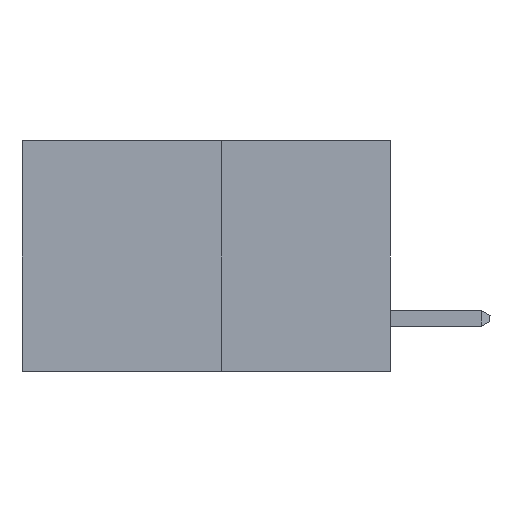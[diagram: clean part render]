
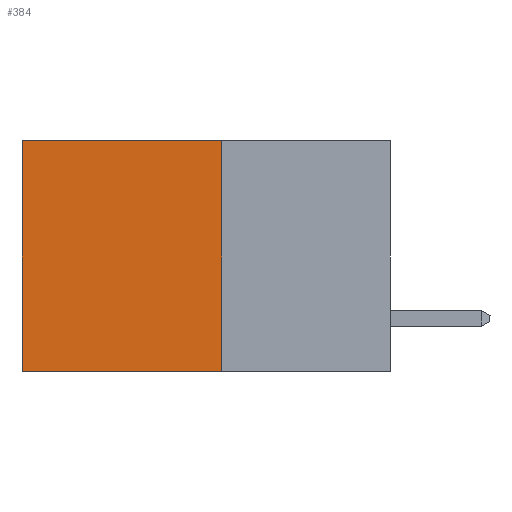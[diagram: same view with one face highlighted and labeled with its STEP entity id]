
A CAD part, left-side view. The second image highlights one B-rep face of the part: STEP entity #384.
In plain terms, the highlighted planar face has unit normal (-1, 0, 0).
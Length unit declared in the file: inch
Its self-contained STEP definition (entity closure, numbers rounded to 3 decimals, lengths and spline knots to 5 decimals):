
#384 = ADVANCED_FACE ( 'NONE', ( #8209 ), #15060, .F. ) ;
#735 = CARTESIAN_POINT ( 'NONE',  ( 0.277, 0.27, -0.37 ) ) ;
#890 = DIRECTION ( 'NONE',  ( 0., 0., -1. ) ) ;
#960 = DIRECTION ( 'NONE',  ( 0., 0., -1. ) ) ;
#1095 = CARTESIAN_POINT ( 'NONE',  ( 0.277, 0.59, -0.37 ) ) ;
#1573 = VERTEX_POINT ( 'NONE', #7489 ) ;
#2374 = LINE ( 'NONE', #735, #22491 ) ;
#2437 = VECTOR ( 'NONE', #17812, 39.37008 ) ;
#3550 = LINE ( 'NONE', #10605, #24242 ) ;
#4259 = VERTEX_POINT ( 'NONE', #1095 ) ;
#4601 = CARTESIAN_POINT ( 'NONE',  ( 0.277, 0.27, 0. ) ) ;
#6029 = CARTESIAN_POINT ( 'NONE',  ( 0.277, 0.27, 0. ) ) ;
#6685 = CARTESIAN_POINT ( 'NONE',  ( 0.277, 0.27, -0.37 ) ) ;
#7489 = CARTESIAN_POINT ( 'NONE',  ( 0.277, 0.59, 0. ) ) ;
#7529 = DIRECTION ( 'NONE',  ( 0., 0., -1. ) ) ;
#7955 = DIRECTION ( 'NONE',  ( 1., 0., 0. ) ) ;
#8033 = ORIENTED_EDGE ( 'NONE', *, *, #11946, .F. ) ;
#8209 = FACE_OUTER_BOUND ( 'NONE', #15707, .T. ) ;
#8269 = EDGE_CURVE ( 'NONE', #14521, #11297, #17312, .T. ) ;
#9212 = ORIENTED_EDGE ( 'NONE', *, *, #19002, .T. ) ;
#10549 = CARTESIAN_POINT ( 'NONE',  ( 0.277, 0.27, -0.37 ) ) ;
#10605 = CARTESIAN_POINT ( 'NONE',  ( 0.277, 0.59, -0.37 ) ) ;
#11297 = VERTEX_POINT ( 'NONE', #6685 ) ;
#11367 = VECTOR ( 'NONE', #890, 39.37008 ) ;
#11946 = EDGE_CURVE ( 'NONE', #11297, #4259, #2374, .T. ) ;
#13365 = ORIENTED_EDGE ( 'NONE', *, *, #15881, .T. ) ;
#14515 = DIRECTION ( 'NONE',  ( 0., 1., 0. ) ) ;
#14521 = VERTEX_POINT ( 'NONE', #4601 ) ;
#15060 = PLANE ( 'NONE',  #25097 ) ;
#15707 = EDGE_LOOP ( 'NONE', ( #13365, #8033, #18260, #9212 ) ) ;
#15881 = EDGE_CURVE ( 'NONE', #1573, #4259, #3550, .T. ) ;
#17312 = LINE ( 'NONE', #10549, #11367 ) ;
#17812 = DIRECTION ( 'NONE',  ( 0., 1., 0. ) ) ;
#18089 = LINE ( 'NONE', #6029, #2437 ) ;
#18260 = ORIENTED_EDGE ( 'NONE', *, *, #8269, .F. ) ;
#19002 = EDGE_CURVE ( 'NONE', #14521, #1573, #18089, .T. ) ;
#19086 = CARTESIAN_POINT ( 'NONE',  ( 0.277, 0.27, -0.37 ) ) ;
#22491 = VECTOR ( 'NONE', #14515, 39.37008 ) ;
#24242 = VECTOR ( 'NONE', #960, 39.37008 ) ;
#25097 = AXIS2_PLACEMENT_3D ( 'NONE', #19086, #7955, #7529 ) ;
